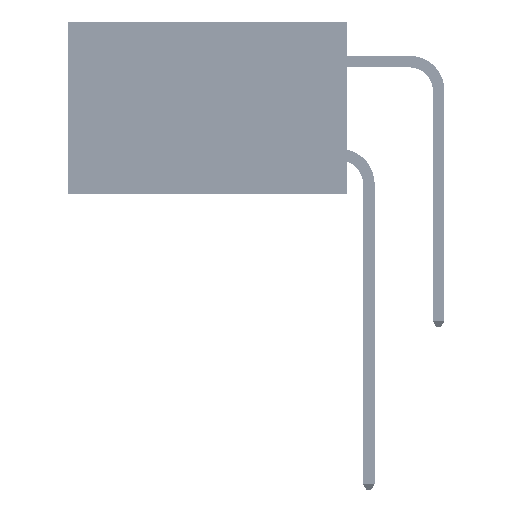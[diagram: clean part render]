
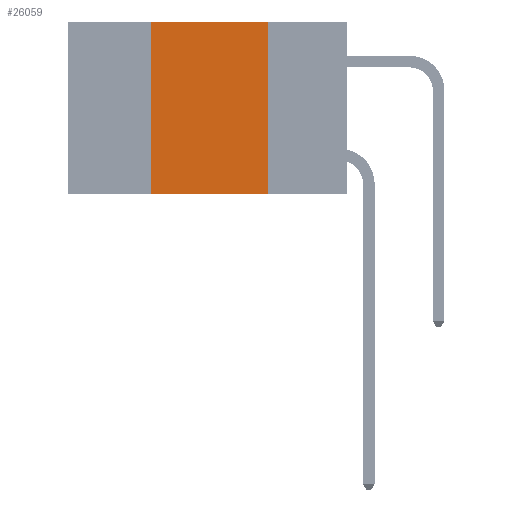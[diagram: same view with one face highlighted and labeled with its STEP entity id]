
A CAD part, left-side view. The second image highlights one B-rep face of the part: STEP entity #26059.
In plain terms, the highlighted planar face has unit normal (-1, 0, 0).
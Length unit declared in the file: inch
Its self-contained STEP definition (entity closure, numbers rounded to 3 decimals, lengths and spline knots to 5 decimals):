
#6 = EDGE_CURVE ( 'NONE', #15290, #13687, #14985, .T. ) ;
#307 = CARTESIAN_POINT ( 'NONE',  ( 0., 0.6, 0. ) ) ;
#2632 = DIRECTION ( 'NONE',  ( 0., 0., -1. ) ) ;
#2854 = CARTESIAN_POINT ( 'NONE',  ( 0., 0.6, 0. ) ) ;
#3207 = DIRECTION ( 'NONE',  ( 0., 0., 1. ) ) ;
#8265 = CARTESIAN_POINT ( 'NONE',  ( 0., 0.6, -0.37 ) ) ;
#8523 = CARTESIAN_POINT ( 'NONE',  ( 0., 0.42, 0. ) ) ;
#8586 = EDGE_LOOP ( 'NONE', ( #27704, #47079, #27542, #40746 ) ) ;
#10550 = LINE ( 'NONE', #34243, #35802 ) ;
#13687 = VERTEX_POINT ( 'NONE', #22531 ) ;
#14985 = LINE ( 'NONE', #8265, #47140 ) ;
#15290 = VERTEX_POINT ( 'NONE', #18143 ) ;
#16587 = DIRECTION ( 'NONE',  ( 0., -1., 0. ) ) ;
#18097 = VERTEX_POINT ( 'NONE', #35917 ) ;
#18143 = CARTESIAN_POINT ( 'NONE',  ( 0., 0.42, -0.37 ) ) ;
#18421 = VECTOR ( 'NONE', #43630, 39.37008 ) ;
#18611 = EDGE_CURVE ( 'NONE', #46527, #18097, #24727, .T. ) ;
#19735 = FACE_OUTER_BOUND ( 'NONE', #8586, .T. ) ;
#22531 = CARTESIAN_POINT ( 'NONE',  ( 0., 0.17, -0.37 ) ) ;
#24727 = LINE ( 'NONE', #2854, #18421 ) ;
#26059 = ADVANCED_FACE ( 'NONE', ( #19735 ), #49241, .F. ) ;
#27542 = ORIENTED_EDGE ( 'NONE', *, *, #28861, .F. ) ;
#27704 = ORIENTED_EDGE ( 'NONE', *, *, #44666, .F. ) ;
#28591 = DIRECTION ( 'NONE',  ( 1., 0., 0. ) ) ;
#28861 = EDGE_CURVE ( 'NONE', #15290, #46527, #43564, .T. ) ;
#32133 = VECTOR ( 'NONE', #3207, 39.37008 ) ;
#34243 = CARTESIAN_POINT ( 'NONE',  ( 0., 0.17, 0. ) ) ;
#35677 = CARTESIAN_POINT ( 'NONE',  ( 0., 0.42, 0. ) ) ;
#35802 = VECTOR ( 'NONE', #2632, 39.37008 ) ;
#35917 = CARTESIAN_POINT ( 'NONE',  ( 0., 0.17, 0. ) ) ;
#37253 = AXIS2_PLACEMENT_3D ( 'NONE', #307, #28591, #45027 ) ;
#40746 = ORIENTED_EDGE ( 'NONE', *, *, #6, .T. ) ;
#43564 = LINE ( 'NONE', #35677, #32133 ) ;
#43630 = DIRECTION ( 'NONE',  ( 0., -1., 0. ) ) ;
#44666 = EDGE_CURVE ( 'NONE', #18097, #13687, #10550, .T. ) ;
#45027 = DIRECTION ( 'NONE',  ( 0., 0., -1. ) ) ;
#46527 = VERTEX_POINT ( 'NONE', #8523 ) ;
#47079 = ORIENTED_EDGE ( 'NONE', *, *, #18611, .F. ) ;
#47140 = VECTOR ( 'NONE', #16587, 39.37008 ) ;
#49241 = PLANE ( 'NONE',  #37253 ) ;
